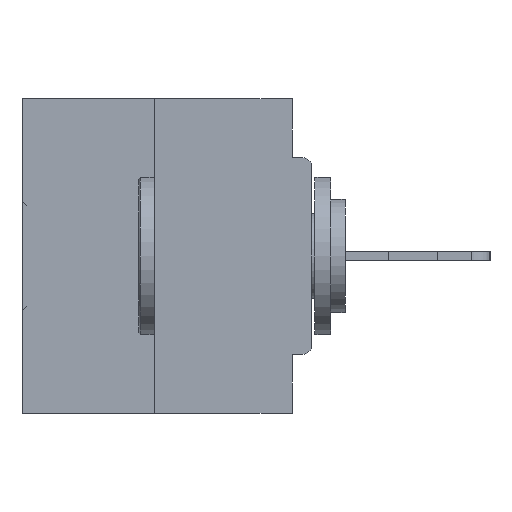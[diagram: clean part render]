
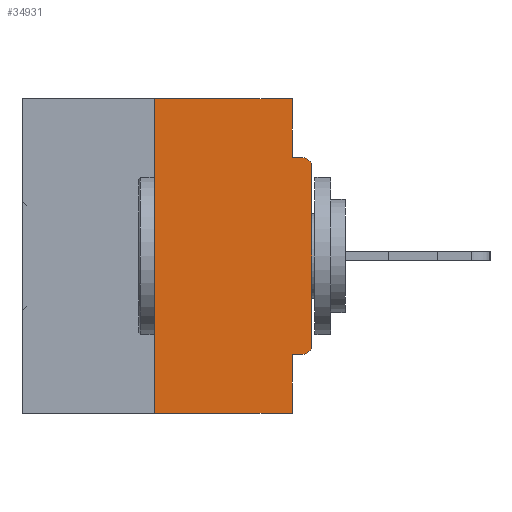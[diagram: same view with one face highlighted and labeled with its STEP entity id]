
A CAD part, left-side view. The second image highlights one B-rep face of the part: STEP entity #34931.
In plain terms, the highlighted planar face has unit normal (-1, 0, 0).
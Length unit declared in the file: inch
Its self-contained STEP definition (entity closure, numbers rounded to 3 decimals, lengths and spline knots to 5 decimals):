
#1760 = EDGE_CURVE ( 'NONE', #3278, #23027, #17480, .T. ) ;
#2273 = FACE_OUTER_BOUND ( 'NONE', #7180, .T. ) ;
#3278 = VERTEX_POINT ( 'NONE', #33496 ) ;
#3294 = VERTEX_POINT ( 'NONE', #30627 ) ;
#4283 = VECTOR ( 'NONE', #25456, 39.37008 ) ;
#4537 = CARTESIAN_POINT ( 'NONE',  ( 0., 0.46, 0. ) ) ;
#5524 = ORIENTED_EDGE ( 'NONE', *, *, #20789, .T. ) ;
#5647 = CARTESIAN_POINT ( 'NONE',  ( 0., 0.46, 0. ) ) ;
#6627 = DIRECTION ( 'NONE',  ( 0., 1., 0. ) ) ;
#6755 = CARTESIAN_POINT ( 'NONE',  ( 0., 0., -0.4065 ) ) ;
#7180 = EDGE_LOOP ( 'NONE', ( #22529, #36833, #22706, #32868, #34638, #33329, #35048, #5524, #11859, #8453 ) ) ;
#7229 = LINE ( 'NONE', #16199, #4283 ) ;
#7408 = DIRECTION ( 'NONE',  ( 0., 0., -1. ) ) ;
#7495 = AXIS2_PLACEMENT_3D ( 'NONE', #4537, #29471, #19795 ) ;
#7653 = DIRECTION ( 'NONE',  ( 0., 0., -1. ) ) ;
#8453 = ORIENTED_EDGE ( 'NONE', *, *, #36021, .F. ) ;
#9867 = VECTOR ( 'NONE', #35058, 39.37008 ) ;
#10120 = LINE ( 'NONE', #5647, #29093 ) ;
#10527 = CARTESIAN_POINT ( 'NONE',  ( 0., 0.015, -0.0935 ) ) ;
#10683 = DIRECTION ( 'NONE',  ( 0., 0., -1. ) ) ;
#10896 = AXIS2_PLACEMENT_3D ( 'NONE', #29754, #32887, #10683 ) ;
#11859 = ORIENTED_EDGE ( 'NONE', *, *, #18616, .F. ) ;
#12117 = CARTESIAN_POINT ( 'NONE',  ( 0., 0.25, -0.5 ) ) ;
#12119 = VERTEX_POINT ( 'NONE', #17670 ) ;
#12367 = EDGE_CURVE ( 'NONE', #23027, #12119, #18132, .T. ) ;
#12662 = EDGE_CURVE ( 'NONE', #24677, #32654, #15674, .T. ) ;
#12962 = LINE ( 'NONE', #35589, #14469 ) ;
#13637 = VERTEX_POINT ( 'NONE', #25610 ) ;
#14469 = VECTOR ( 'NONE', #7408, 39.37008 ) ;
#14519 = VECTOR ( 'NONE', #7653, 39.37008 ) ;
#14976 = CARTESIAN_POINT ( 'NONE',  ( 0., 0.25, 0. ) ) ;
#15052 = EDGE_CURVE ( 'NONE', #24677, #32726, #7229, .T. ) ;
#15122 = DIRECTION ( 'NONE',  ( 0., -1., 0. ) ) ;
#15674 = LINE ( 'NONE', #21130, #23526 ) ;
#16199 = CARTESIAN_POINT ( 'NONE',  ( 0., 0.25, 0. ) ) ;
#16565 = VECTOR ( 'NONE', #25046, 39.37008 ) ;
#17480 = CIRCLE ( 'NONE', #10896, 0.015 ) ;
#17670 = CARTESIAN_POINT ( 'NONE',  ( 0., 0., -0.1085 ) ) ;
#18132 = LINE ( 'NONE', #19089, #9867 ) ;
#18616 = EDGE_CURVE ( 'NONE', #3294, #35298, #34610, .T. ) ;
#19034 = CARTESIAN_POINT ( 'NONE',  ( 0., 0., -0.3915 ) ) ;
#19089 = CARTESIAN_POINT ( 'NONE',  ( 0., 0., 0. ) ) ;
#19118 = PLANE ( 'NONE',  #7495 ) ;
#19795 = DIRECTION ( 'NONE',  ( 0., 0., -1. ) ) ;
#20311 = DIRECTION ( 'NONE',  ( 0., 0., -1. ) ) ;
#20789 = EDGE_CURVE ( 'NONE', #12119, #35298, #36435, .T. ) ;
#21130 = CARTESIAN_POINT ( 'NONE',  ( 0., 0.46, -0.5 ) ) ;
#21334 = DIRECTION ( 'NONE',  ( 0., -1., 0. ) ) ;
#22529 = ORIENTED_EDGE ( 'NONE', *, *, #34760, .F. ) ;
#22706 = ORIENTED_EDGE ( 'NONE', *, *, #12662, .T. ) ;
#23027 = VERTEX_POINT ( 'NONE', #19034 ) ;
#23526 = VECTOR ( 'NONE', #15122, 39.37008 ) ;
#23694 = VECTOR ( 'NONE', #6627, 39.37008 ) ;
#24677 = VERTEX_POINT ( 'NONE', #12117 ) ;
#24731 = LINE ( 'NONE', #35566, #14519 ) ;
#25046 = DIRECTION ( 'NONE',  ( 0., -1., 0. ) ) ;
#25456 = DIRECTION ( 'NONE',  ( 0., 0., 1. ) ) ;
#25557 = CARTESIAN_POINT ( 'NONE',  ( 0., 0.031, -0.4065 ) ) ;
#25610 = CARTESIAN_POINT ( 'NONE',  ( 0., 0.031, 0. ) ) ;
#26192 = EDGE_CURVE ( 'NONE', #39785, #32654, #24731, .T. ) ;
#28438 = CARTESIAN_POINT ( 'NONE',  ( 0., 0., -0.0935 ) ) ;
#29093 = VECTOR ( 'NONE', #21334, 39.37008 ) ;
#29471 = DIRECTION ( 'NONE',  ( 1., 0., 0. ) ) ;
#29634 = EDGE_CURVE ( 'NONE', #3278, #39785, #39245, .T. ) ;
#29754 = CARTESIAN_POINT ( 'NONE',  ( 0., 0.015, -0.3915 ) ) ;
#30627 = CARTESIAN_POINT ( 'NONE',  ( 0., 0.031, -0.0935 ) ) ;
#32654 = VERTEX_POINT ( 'NONE', #33653 ) ;
#32726 = VERTEX_POINT ( 'NONE', #14976 ) ;
#32868 = ORIENTED_EDGE ( 'NONE', *, *, #26192, .F. ) ;
#32887 = DIRECTION ( 'NONE',  ( -1., 0., 0. ) ) ;
#32948 = AXIS2_PLACEMENT_3D ( 'NONE', #32994, #35603, #20311 ) ;
#32994 = CARTESIAN_POINT ( 'NONE',  ( 0., 0.015, -0.1085 ) ) ;
#33329 = ORIENTED_EDGE ( 'NONE', *, *, #1760, .T. ) ;
#33496 = CARTESIAN_POINT ( 'NONE',  ( 0., 0.015, -0.4065 ) ) ;
#33653 = CARTESIAN_POINT ( 'NONE',  ( 0., 0.031, -0.5 ) ) ;
#34610 = LINE ( 'NONE', #28438, #16565 ) ;
#34638 = ORIENTED_EDGE ( 'NONE', *, *, #29634, .F. ) ;
#34760 = EDGE_CURVE ( 'NONE', #32726, #13637, #10120, .T. ) ;
#34931 = ADVANCED_FACE ( 'NONE', ( #2273 ), #19118, .F. ) ;
#35048 = ORIENTED_EDGE ( 'NONE', *, *, #12367, .T. ) ;
#35058 = DIRECTION ( 'NONE',  ( 0., 0., 1. ) ) ;
#35298 = VERTEX_POINT ( 'NONE', #10527 ) ;
#35566 = CARTESIAN_POINT ( 'NONE',  ( 0., 0.031, -0.5 ) ) ;
#35589 = CARTESIAN_POINT ( 'NONE',  ( 0., 0.031, 0. ) ) ;
#35603 = DIRECTION ( 'NONE',  ( -1., 0., 0. ) ) ;
#36021 = EDGE_CURVE ( 'NONE', #13637, #3294, #12962, .T. ) ;
#36435 = CIRCLE ( 'NONE', #32948, 0.015 ) ;
#36833 = ORIENTED_EDGE ( 'NONE', *, *, #15052, .F. ) ;
#39245 = LINE ( 'NONE', #6755, #23694 ) ;
#39785 = VERTEX_POINT ( 'NONE', #25557 ) ;
